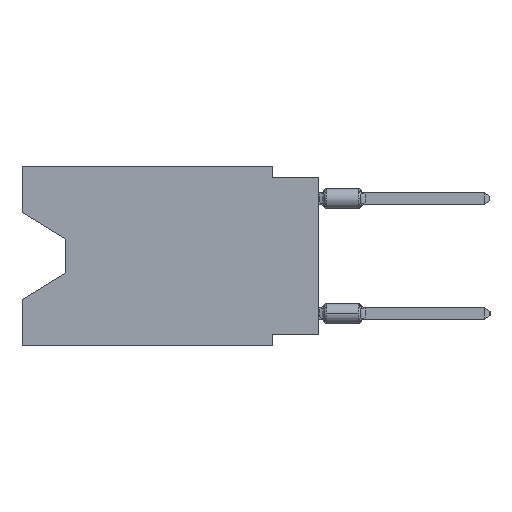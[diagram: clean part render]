
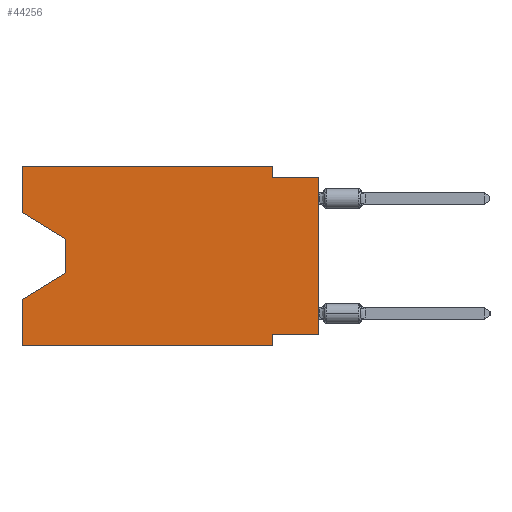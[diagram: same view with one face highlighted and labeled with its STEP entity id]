
A CAD part, left-side view. The second image highlights one B-rep face of the part: STEP entity #44256.
In plain terms, the highlighted planar face has unit normal (-1, 0, 0).
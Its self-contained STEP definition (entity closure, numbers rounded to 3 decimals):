
#174 = ORIENTED_EDGE ( 'NONE', *, *, #23360, .F. ) ;
#433 = VERTEX_POINT ( 'NONE', #62690 ) ;
#876 = VECTOR ( 'NONE', #1524, 1000. ) ;
#1150 = CARTESIAN_POINT ( 'NONE',  ( 0., 2.54, -9.271 ) ) ;
#1189 = EDGE_CURVE ( 'NONE', #433, #34642, #45509, .T. ) ;
#1524 = DIRECTION ( 'NONE',  ( 0., 1., 0. ) ) ;
#2319 = DIRECTION ( 'NONE',  ( 0., -1., 0. ) ) ;
#2655 = VERTEX_POINT ( 'NONE', #24449 ) ;
#3766 = CARTESIAN_POINT ( 'NONE',  ( 0., 16.383, 0. ) ) ;
#4420 = ORIENTED_EDGE ( 'NONE', *, *, #64697, .T. ) ;
#4558 = EDGE_CURVE ( 'NONE', #34642, #28105, #64223, .T. ) ;
#4643 = DIRECTION ( 'NONE',  ( 0., 0., 1. ) ) ;
#5066 = VERTEX_POINT ( 'NONE', #54299 ) ;
#5150 = CARTESIAN_POINT ( 'NONE',  ( 0., 0., -9.271 ) ) ;
#5393 = EDGE_CURVE ( 'NONE', #2655, #51142, #22410, .T. ) ;
#5447 = VECTOR ( 'NONE', #53431, 1000. ) ;
#5557 = ORIENTED_EDGE ( 'NONE', *, *, #27330, .F. ) ;
#5987 = DIRECTION ( 'NONE',  ( 0., -1., 0. ) ) ;
#6517 = VERTEX_POINT ( 'NONE', #1150 ) ;
#8219 = ORIENTED_EDGE ( 'NONE', *, *, #1189, .F. ) ;
#8225 = DIRECTION ( 'NONE',  ( 0., 0.855, -0.519 ) ) ;
#9100 = VECTOR ( 'NONE', #8225, 1000. ) ;
#9467 = DIRECTION ( 'NONE',  ( 0., 0., -1. ) ) ;
#9605 = CARTESIAN_POINT ( 'NONE',  ( 0., 2.54, -9.906 ) ) ;
#9874 = CARTESIAN_POINT ( 'NONE',  ( 0., 16.383, 0. ) ) ;
#11319 = VECTOR ( 'NONE', #4643, 1000. ) ;
#11396 = CARTESIAN_POINT ( 'NONE',  ( 0., 16.383, 0. ) ) ;
#11700 = CARTESIAN_POINT ( 'NONE',  ( 0., 2.54, 0. ) ) ;
#12512 = CARTESIAN_POINT ( 'NONE',  ( 0., 13.97, -5.893 ) ) ;
#12593 = CARTESIAN_POINT ( 'NONE',  ( 0., 2.54, -9.906 ) ) ;
#12967 = VECTOR ( 'NONE', #39287, 1000. ) ;
#13550 = DIRECTION ( 'NONE',  ( 0., 0., -1. ) ) ;
#14387 = CARTESIAN_POINT ( 'NONE',  ( 0., 16.383, 0. ) ) ;
#16328 = CARTESIAN_POINT ( 'NONE',  ( 0., 16.383, -2.546 ) ) ;
#18196 = DIRECTION ( 'NONE',  ( 0., 0., 1. ) ) ;
#18308 = EDGE_LOOP ( 'NONE', ( #54190, #20740, #52246, #5557, #58131, #46306, #39247, #4420, #174, #40972, #8219, #41259 ) ) ;
#18790 = CARTESIAN_POINT ( 'NONE',  ( 0., 0., 0. ) ) ;
#20224 = EDGE_CURVE ( 'NONE', #44260, #2655, #59029, .T. ) ;
#20740 = ORIENTED_EDGE ( 'NONE', *, *, #5393, .T. ) ;
#22410 = LINE ( 'NONE', #62445, #40308 ) ;
#22910 = CARTESIAN_POINT ( 'NONE',  ( 0., 16.383, -7.36 ) ) ;
#23360 = EDGE_CURVE ( 'NONE', #28105, #35986, #46938, .T. ) ;
#24020 = DIRECTION ( 'NONE',  ( 0., 0., -1. ) ) ;
#24449 = CARTESIAN_POINT ( 'NONE',  ( 0., 13.97, -4.013 ) ) ;
#25348 = VECTOR ( 'NONE', #5987, 1000. ) ;
#25663 = LINE ( 'NONE', #45669, #25348 ) ;
#25833 = FACE_OUTER_BOUND ( 'NONE', #18308, .T. ) ;
#25997 = VECTOR ( 'NONE', #18196, 1000. ) ;
#26166 = EDGE_CURVE ( 'NONE', #51142, #53821, #63665, .T. ) ;
#27330 = EDGE_CURVE ( 'NONE', #40767, #53821, #48593, .T. ) ;
#28101 = CARTESIAN_POINT ( 'NONE',  ( 0., 16.383, -9.906 ) ) ;
#28105 = VERTEX_POINT ( 'NONE', #53671 ) ;
#29743 = EDGE_CURVE ( 'NONE', #44260, #433, #33916, .T. ) ;
#31388 = CARTESIAN_POINT ( 'NONE',  ( 0., 13.97, -5.893 ) ) ;
#31757 = VECTOR ( 'NONE', #2319, 1000. ) ;
#33855 = EDGE_CURVE ( 'NONE', #5066, #6517, #55988, .T. ) ;
#33916 = LINE ( 'NONE', #3766, #25997 ) ;
#34371 = DIRECTION ( 'NONE',  ( 1., 0., 0. ) ) ;
#34642 = VERTEX_POINT ( 'NONE', #11700 ) ;
#35968 = CARTESIAN_POINT ( 'NONE',  ( 0., 0., -0.635 ) ) ;
#35986 = VERTEX_POINT ( 'NONE', #35968 ) ;
#38069 = EDGE_CURVE ( 'NONE', #40767, #43103, #25663, .T. ) ;
#38198 = VECTOR ( 'NONE', #24020, 1000. ) ;
#39247 = ORIENTED_EDGE ( 'NONE', *, *, #33855, .F. ) ;
#39287 = DIRECTION ( 'NONE',  ( 0., 0., -1. ) ) ;
#40308 = VECTOR ( 'NONE', #13550, 1000. ) ;
#40767 = VERTEX_POINT ( 'NONE', #28101 ) ;
#40972 = ORIENTED_EDGE ( 'NONE', *, *, #4558, .F. ) ;
#41259 = ORIENTED_EDGE ( 'NONE', *, *, #29743, .F. ) ;
#42649 = CARTESIAN_POINT ( 'NONE',  ( 0., 0., -0.635 ) ) ;
#43103 = VERTEX_POINT ( 'NONE', #12593 ) ;
#44256 = ADVANCED_FACE ( 'NONE', ( #25833 ), #45847, .F. ) ;
#44260 = VERTEX_POINT ( 'NONE', #16328 ) ;
#45509 = LINE ( 'NONE', #11396, #51867 ) ;
#45669 = CARTESIAN_POINT ( 'NONE',  ( 0., 16.383, -9.906 ) ) ;
#45847 = PLANE ( 'NONE',  #51881 ) ;
#46306 = ORIENTED_EDGE ( 'NONE', *, *, #63417, .F. ) ;
#46938 = LINE ( 'NONE', #42649, #31757 ) ;
#48151 = CARTESIAN_POINT ( 'NONE',  ( 0., 2.54, 0. ) ) ;
#48519 = CARTESIAN_POINT ( 'NONE',  ( 0., 16.383, -2.546 ) ) ;
#48593 = LINE ( 'NONE', #9874, #11319 ) ;
#48967 = LINE ( 'NONE', #9605, #38198 ) ;
#48977 = LINE ( 'NONE', #18790, #49860 ) ;
#49860 = VECTOR ( 'NONE', #59488, 1000. ) ;
#51142 = VERTEX_POINT ( 'NONE', #31388 ) ;
#51713 = DIRECTION ( 'NONE',  ( 0., -1., 0. ) ) ;
#51867 = VECTOR ( 'NONE', #51713, 1000. ) ;
#51881 = AXIS2_PLACEMENT_3D ( 'NONE', #14387, #34371, #9467 ) ;
#52246 = ORIENTED_EDGE ( 'NONE', *, *, #26166, .T. ) ;
#53431 = DIRECTION ( 'NONE',  ( 0., -0.855, -0.519 ) ) ;
#53671 = CARTESIAN_POINT ( 'NONE',  ( 0., 2.54, -0.635 ) ) ;
#53821 = VERTEX_POINT ( 'NONE', #22910 ) ;
#54190 = ORIENTED_EDGE ( 'NONE', *, *, #20224, .T. ) ;
#54299 = CARTESIAN_POINT ( 'NONE',  ( 0., 0., -9.271 ) ) ;
#55988 = LINE ( 'NONE', #5150, #876 ) ;
#58131 = ORIENTED_EDGE ( 'NONE', *, *, #38069, .T. ) ;
#59029 = LINE ( 'NONE', #48519, #5447 ) ;
#59488 = DIRECTION ( 'NONE',  ( 0., 0., 1. ) ) ;
#62445 = CARTESIAN_POINT ( 'NONE',  ( 0., 13.97, -4.013 ) ) ;
#62690 = CARTESIAN_POINT ( 'NONE',  ( 0., 16.383, 0. ) ) ;
#63417 = EDGE_CURVE ( 'NONE', #6517, #43103, #48967, .T. ) ;
#63665 = LINE ( 'NONE', #12512, #9100 ) ;
#64223 = LINE ( 'NONE', #48151, #12967 ) ;
#64697 = EDGE_CURVE ( 'NONE', #5066, #35986, #48977, .T. ) ;
